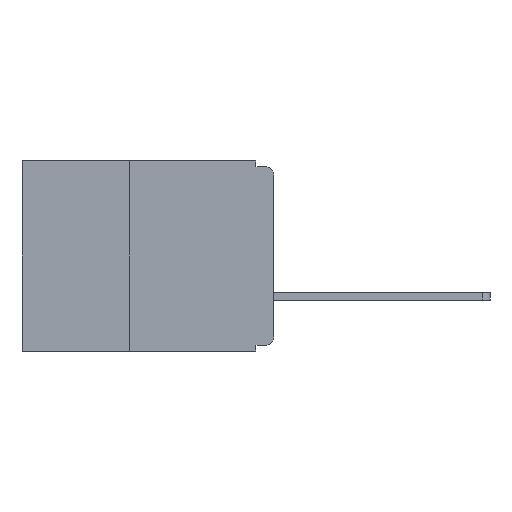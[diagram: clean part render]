
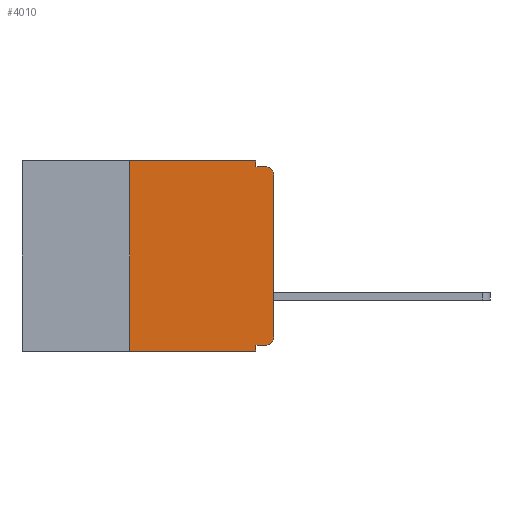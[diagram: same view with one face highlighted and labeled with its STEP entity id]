
A CAD part, left-side view. The second image highlights one B-rep face of the part: STEP entity #4010.
In plain terms, the highlighted planar face has unit normal (-1, 0, 0).
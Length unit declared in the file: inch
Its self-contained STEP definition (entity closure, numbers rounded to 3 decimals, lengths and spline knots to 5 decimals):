
#161 = CARTESIAN_POINT ( 'NONE',  ( 0., 0., 0. ) ) ;
#304 = VECTOR ( 'NONE', #20590, 39.37008 ) ;
#392 = ORIENTED_EDGE ( 'NONE', *, *, #22961, .T. ) ;
#513 = VERTEX_POINT ( 'NONE', #21367 ) ;
#612 = CIRCLE ( 'NONE', #5443, 0.015 ) ;
#711 = ORIENTED_EDGE ( 'NONE', *, *, #910, .F. ) ;
#910 = EDGE_CURVE ( 'NONE', #6898, #16722, #11971, .T. ) ;
#1014 = ORIENTED_EDGE ( 'NONE', *, *, #19003, .F. ) ;
#1225 = EDGE_LOOP ( 'NONE', ( #2651, #392, #711, #1014, #1865, #3066, #4032, #6824, #7036, #8094 ) ) ;
#1400 = VERTEX_POINT ( 'NONE', #8431 ) ;
#1865 = ORIENTED_EDGE ( 'NONE', *, *, #8919, .F. ) ;
#2013 = EDGE_CURVE ( 'NONE', #1400, #8742, #22388, .T. ) ;
#2651 = ORIENTED_EDGE ( 'NONE', *, *, #26861, .T. ) ;
#2850 = VECTOR ( 'NONE', #6821, 39.37008 ) ;
#3066 = ORIENTED_EDGE ( 'NONE', *, *, #21758, .F. ) ;
#3156 = EDGE_CURVE ( 'NONE', #15772, #8742, #16276, .T. ) ;
#3511 = CARTESIAN_POINT ( 'NONE',  ( 0., 0., -0.32 ) ) ;
#4010 = ADVANCED_FACE ( 'NONE', ( #16227 ), #23766, .F. ) ;
#4032 = ORIENTED_EDGE ( 'NONE', *, *, #2013, .T. ) ;
#5443 = AXIS2_PLACEMENT_3D ( 'NONE', #21942, #9078, #24107 ) ;
#5720 = DIRECTION ( 'NONE',  ( 0., 1., 0. ) ) ;
#6014 = CARTESIAN_POINT ( 'NONE',  ( 0., 0.031, 0. ) ) ;
#6476 = DIRECTION ( 'NONE',  ( 0., -1., 0. ) ) ;
#6560 = CARTESIAN_POINT ( 'NONE',  ( 0., 0.015, -0.01 ) ) ;
#6563 = DIRECTION ( 'NONE',  ( 0., 0., 1. ) ) ;
#6821 = DIRECTION ( 'NONE',  ( 0., 0., 1. ) ) ;
#6824 = ORIENTED_EDGE ( 'NONE', *, *, #3156, .F. ) ;
#6862 = DIRECTION ( 'NONE',  ( 0., -1., 0. ) ) ;
#6898 = VERTEX_POINT ( 'NONE', #10320 ) ;
#7036 = ORIENTED_EDGE ( 'NONE', *, *, #13549, .F. ) ;
#7408 = VECTOR ( 'NONE', #23272, 39.37008 ) ;
#7783 = LINE ( 'NONE', #15077, #24264 ) ;
#8082 = CIRCLE ( 'NONE', #21387, 0.015 ) ;
#8094 = ORIENTED_EDGE ( 'NONE', *, *, #18841, .T. ) ;
#8431 = CARTESIAN_POINT ( 'NONE',  ( 0., 0.25, -0.33 ) ) ;
#8742 = VERTEX_POINT ( 'NONE', #12275 ) ;
#8919 = EDGE_CURVE ( 'NONE', #513, #14859, #7783, .T. ) ;
#9078 = DIRECTION ( 'NONE',  ( -1., 0., 0. ) ) ;
#9634 = LINE ( 'NONE', #10953, #25372 ) ;
#9765 = DIRECTION ( 'NONE',  ( -1., 0., 0. ) ) ;
#10320 = CARTESIAN_POINT ( 'NONE',  ( 0., 0.031, -0.01 ) ) ;
#10953 = CARTESIAN_POINT ( 'NONE',  ( 0., 0.25, -0.33 ) ) ;
#11066 = CARTESIAN_POINT ( 'NONE',  ( 0., 0.437, -0.33 ) ) ;
#11971 = LINE ( 'NONE', #20404, #304 ) ;
#12275 = CARTESIAN_POINT ( 'NONE',  ( 0., 0.031, -0.33 ) ) ;
#12299 = CARTESIAN_POINT ( 'NONE',  ( 0., 0.015, -0.32 ) ) ;
#13549 = EDGE_CURVE ( 'NONE', #18984, #15772, #27450, .T. ) ;
#14450 = LINE ( 'NONE', #161, #2850 ) ;
#14859 = VERTEX_POINT ( 'NONE', #15033 ) ;
#15033 = CARTESIAN_POINT ( 'NONE',  ( 0., 0.031, 0. ) ) ;
#15077 = CARTESIAN_POINT ( 'NONE',  ( 0., 0.437, 0. ) ) ;
#15772 = VERTEX_POINT ( 'NONE', #20418 ) ;
#16136 = VECTOR ( 'NONE', #5720, 39.37008 ) ;
#16227 = FACE_OUTER_BOUND ( 'NONE', #1225, .T. ) ;
#16276 = LINE ( 'NONE', #23335, #21994 ) ;
#16665 = VECTOR ( 'NONE', #6862, 39.37008 ) ;
#16722 = VERTEX_POINT ( 'NONE', #6560 ) ;
#17150 = CARTESIAN_POINT ( 'NONE',  ( 0., 0., -0.305 ) ) ;
#18548 = VERTEX_POINT ( 'NONE', #17150 ) ;
#18831 = LINE ( 'NONE', #6014, #7408 ) ;
#18841 = EDGE_CURVE ( 'NONE', #18984, #18548, #8082, .T. ) ;
#18984 = VERTEX_POINT ( 'NONE', #12299 ) ;
#19003 = EDGE_CURVE ( 'NONE', #14859, #6898, #18831, .T. ) ;
#19857 = VERTEX_POINT ( 'NONE', #23871 ) ;
#20404 = CARTESIAN_POINT ( 'NONE',  ( 0., 0., -0.01 ) ) ;
#20418 = CARTESIAN_POINT ( 'NONE',  ( 0., 0.031, -0.32 ) ) ;
#20590 = DIRECTION ( 'NONE',  ( 0., -1., 0. ) ) ;
#21367 = CARTESIAN_POINT ( 'NONE',  ( 0., 0.25, 0. ) ) ;
#21387 = AXIS2_PLACEMENT_3D ( 'NONE', #22608, #9765, #24740 ) ;
#21758 = EDGE_CURVE ( 'NONE', #1400, #513, #9634, .T. ) ;
#21942 = CARTESIAN_POINT ( 'NONE',  ( 0., 0.015, -0.025 ) ) ;
#21994 = VECTOR ( 'NONE', #23596, 39.37008 ) ;
#22388 = LINE ( 'NONE', #11066, #16665 ) ;
#22608 = CARTESIAN_POINT ( 'NONE',  ( 0., 0.015, -0.305 ) ) ;
#22961 = EDGE_CURVE ( 'NONE', #19857, #16722, #612, .T. ) ;
#22997 = DIRECTION ( 'NONE',  ( 0., 0., -1. ) ) ;
#23092 = DIRECTION ( 'NONE',  ( 1., 0., 0. ) ) ;
#23272 = DIRECTION ( 'NONE',  ( 0., 0., -1. ) ) ;
#23335 = CARTESIAN_POINT ( 'NONE',  ( 0., 0.031, -0.33 ) ) ;
#23596 = DIRECTION ( 'NONE',  ( 0., 0., -1. ) ) ;
#23733 = CARTESIAN_POINT ( 'NONE',  ( 0., 0.437, 0. ) ) ;
#23766 = PLANE ( 'NONE',  #26235 ) ;
#23871 = CARTESIAN_POINT ( 'NONE',  ( 0., 0., -0.025 ) ) ;
#24107 = DIRECTION ( 'NONE',  ( 0., 0., -1. ) ) ;
#24264 = VECTOR ( 'NONE', #6476, 39.37008 ) ;
#24740 = DIRECTION ( 'NONE',  ( 0., 0., -1. ) ) ;
#25372 = VECTOR ( 'NONE', #6563, 39.37008 ) ;
#26235 = AXIS2_PLACEMENT_3D ( 'NONE', #23733, #23092, #22997 ) ;
#26861 = EDGE_CURVE ( 'NONE', #18548, #19857, #14450, .T. ) ;
#27450 = LINE ( 'NONE', #3511, #16136 ) ;
